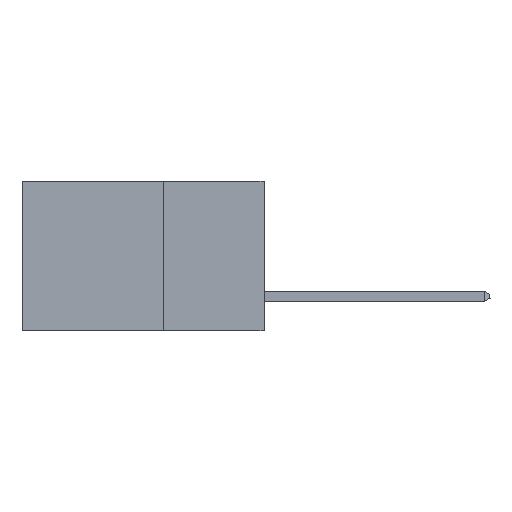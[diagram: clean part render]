
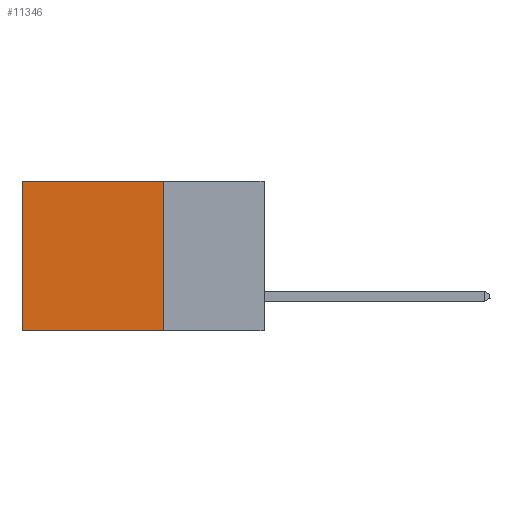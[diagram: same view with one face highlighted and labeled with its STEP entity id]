
A CAD part, left-side view. The second image highlights one B-rep face of the part: STEP entity #11346.
In plain terms, the highlighted planar face has unit normal (-1, 0, 0).
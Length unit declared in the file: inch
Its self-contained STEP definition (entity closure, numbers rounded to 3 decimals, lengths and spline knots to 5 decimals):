
#25 = CARTESIAN_POINT ( 'NONE',  ( 0.298, 0.6, 0. ) ) ;
#143 = VECTOR ( 'NONE', #9984, 39.37008 ) ;
#384 = DIRECTION ( 'NONE',  ( 0., 1., 0. ) ) ;
#591 = PLANE ( 'NONE',  #11244 ) ;
#618 = EDGE_LOOP ( 'NONE', ( #5090, #4862, #12189, #7566 ) ) ;
#678 = EDGE_CURVE ( 'NONE', #3157, #7270, #4547, .T. ) ;
#726 = CARTESIAN_POINT ( 'NONE',  ( 0.298, 0.25, 0. ) ) ;
#1477 = EDGE_CURVE ( 'NONE', #7270, #2345, #1765, .T. ) ;
#1532 = CARTESIAN_POINT ( 'NONE',  ( 0.298, 0.6, 0. ) ) ;
#1658 = CARTESIAN_POINT ( 'NONE',  ( 0.298, 0.25, 0. ) ) ;
#1714 = DIRECTION ( 'NONE',  ( 1., 0., 0. ) ) ;
#1765 = LINE ( 'NONE', #1532, #9516 ) ;
#2345 = VERTEX_POINT ( 'NONE', #7920 ) ;
#3157 = VERTEX_POINT ( 'NONE', #12291 ) ;
#3372 = CARTESIAN_POINT ( 'NONE',  ( 0.298, 0.25, -0.37 ) ) ;
#3457 = CARTESIAN_POINT ( 'NONE',  ( 0.298, 0.25, 0. ) ) ;
#4002 = LINE ( 'NONE', #8566, #6450 ) ;
#4032 = EDGE_CURVE ( 'NONE', #3157, #5004, #8245, .T. ) ;
#4366 = EDGE_CURVE ( 'NONE', #5004, #2345, #4002, .T. ) ;
#4425 = DIRECTION ( 'NONE',  ( 0., 1., 0. ) ) ;
#4547 = LINE ( 'NONE', #3457, #5357 ) ;
#4862 = ORIENTED_EDGE ( 'NONE', *, *, #4366, .F. ) ;
#5004 = VERTEX_POINT ( 'NONE', #3372 ) ;
#5075 = FACE_OUTER_BOUND ( 'NONE', #618, .T. ) ;
#5090 = ORIENTED_EDGE ( 'NONE', *, *, #1477, .T. ) ;
#5357 = VECTOR ( 'NONE', #384, 39.37008 ) ;
#5935 = DIRECTION ( 'NONE',  ( 0., 0., -1. ) ) ;
#6450 = VECTOR ( 'NONE', #4425, 39.37008 ) ;
#7270 = VERTEX_POINT ( 'NONE', #25 ) ;
#7566 = ORIENTED_EDGE ( 'NONE', *, *, #678, .T. ) ;
#7920 = CARTESIAN_POINT ( 'NONE',  ( 0.298, 0.6, -0.37 ) ) ;
#8245 = LINE ( 'NONE', #1658, #143 ) ;
#8566 = CARTESIAN_POINT ( 'NONE',  ( 0.298, 0.25, -0.37 ) ) ;
#9516 = VECTOR ( 'NONE', #10906, 39.37008 ) ;
#9984 = DIRECTION ( 'NONE',  ( 0., 0., -1. ) ) ;
#10906 = DIRECTION ( 'NONE',  ( 0., 0., -1. ) ) ;
#11244 = AXIS2_PLACEMENT_3D ( 'NONE', #726, #1714, #5935 ) ;
#11346 = ADVANCED_FACE ( 'NONE', ( #5075 ), #591, .F. ) ;
#12189 = ORIENTED_EDGE ( 'NONE', *, *, #4032, .F. ) ;
#12291 = CARTESIAN_POINT ( 'NONE',  ( 0.298, 0.25, 0. ) ) ;
